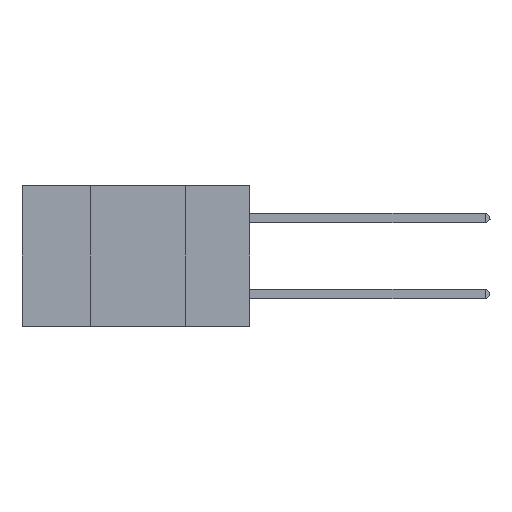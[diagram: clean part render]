
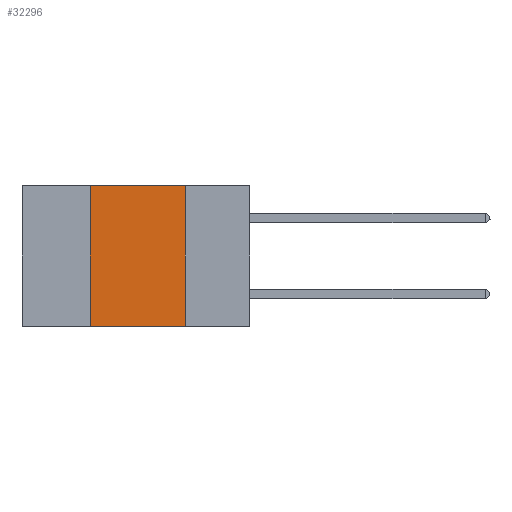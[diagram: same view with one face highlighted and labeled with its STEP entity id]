
A CAD part, left-side view. The second image highlights one B-rep face of the part: STEP entity #32296.
In plain terms, the highlighted planar face has unit normal (-1, 0, 0).
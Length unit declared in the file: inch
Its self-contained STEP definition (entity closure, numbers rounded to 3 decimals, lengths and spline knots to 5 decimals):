
#523 = EDGE_LOOP ( 'NONE', ( #15769, #11180, #16294, #30586 ) ) ;
#2901 = LINE ( 'NONE', #24019, #29472 ) ;
#4941 = DIRECTION ( 'NONE',  ( 0., 0., -1. ) ) ;
#5215 = CARTESIAN_POINT ( 'NONE',  ( 0., 0.42, 0. ) ) ;
#5394 = EDGE_CURVE ( 'NONE', #33980, #13489, #20528, .T. ) ;
#5397 = VECTOR ( 'NONE', #29555, 39.37008 ) ;
#5689 = LINE ( 'NONE', #13650, #25819 ) ;
#8402 = CARTESIAN_POINT ( 'NONE',  ( 0., 0.6, 0. ) ) ;
#11180 = ORIENTED_EDGE ( 'NONE', *, *, #15138, .F. ) ;
#12558 = CARTESIAN_POINT ( 'NONE',  ( 0., 0.6, 0. ) ) ;
#12571 = VERTEX_POINT ( 'NONE', #5215 ) ;
#13489 = VERTEX_POINT ( 'NONE', #15494 ) ;
#13650 = CARTESIAN_POINT ( 'NONE',  ( 0., 0.42, 0. ) ) ;
#14563 = EDGE_CURVE ( 'NONE', #33980, #12571, #5689, .T. ) ;
#15138 = EDGE_CURVE ( 'NONE', #12571, #15322, #32147, .T. ) ;
#15322 = VERTEX_POINT ( 'NONE', #22924 ) ;
#15494 = CARTESIAN_POINT ( 'NONE',  ( 0., 0.17, -0.37 ) ) ;
#15769 = ORIENTED_EDGE ( 'NONE', *, *, #19968, .F. ) ;
#16294 = ORIENTED_EDGE ( 'NONE', *, *, #14563, .F. ) ;
#17715 = AXIS2_PLACEMENT_3D ( 'NONE', #12558, #28665, #4941 ) ;
#18091 = PLANE ( 'NONE',  #17715 ) ;
#19968 = EDGE_CURVE ( 'NONE', #15322, #13489, #2901, .T. ) ;
#20528 = LINE ( 'NONE', #31130, #20545 ) ;
#20545 = VECTOR ( 'NONE', #23309, 39.37008 ) ;
#22046 = CARTESIAN_POINT ( 'NONE',  ( 0., 0.42, -0.37 ) ) ;
#22924 = CARTESIAN_POINT ( 'NONE',  ( 0., 0.17, 0. ) ) ;
#23309 = DIRECTION ( 'NONE',  ( 0., -1., 0. ) ) ;
#23504 = DIRECTION ( 'NONE',  ( 0., 0., -1. ) ) ;
#23532 = DIRECTION ( 'NONE',  ( 0., 0., 1. ) ) ;
#24019 = CARTESIAN_POINT ( 'NONE',  ( 0., 0.17, 0. ) ) ;
#25819 = VECTOR ( 'NONE', #23532, 39.37008 ) ;
#28665 = DIRECTION ( 'NONE',  ( 1., 0., 0. ) ) ;
#29472 = VECTOR ( 'NONE', #23504, 39.37008 ) ;
#29555 = DIRECTION ( 'NONE',  ( 0., -1., 0. ) ) ;
#30586 = ORIENTED_EDGE ( 'NONE', *, *, #5394, .T. ) ;
#31130 = CARTESIAN_POINT ( 'NONE',  ( 0., 0.6, -0.37 ) ) ;
#32147 = LINE ( 'NONE', #8402, #5397 ) ;
#32296 = ADVANCED_FACE ( 'NONE', ( #33700 ), #18091, .F. ) ;
#33700 = FACE_OUTER_BOUND ( 'NONE', #523, .T. ) ;
#33980 = VERTEX_POINT ( 'NONE', #22046 ) ;
